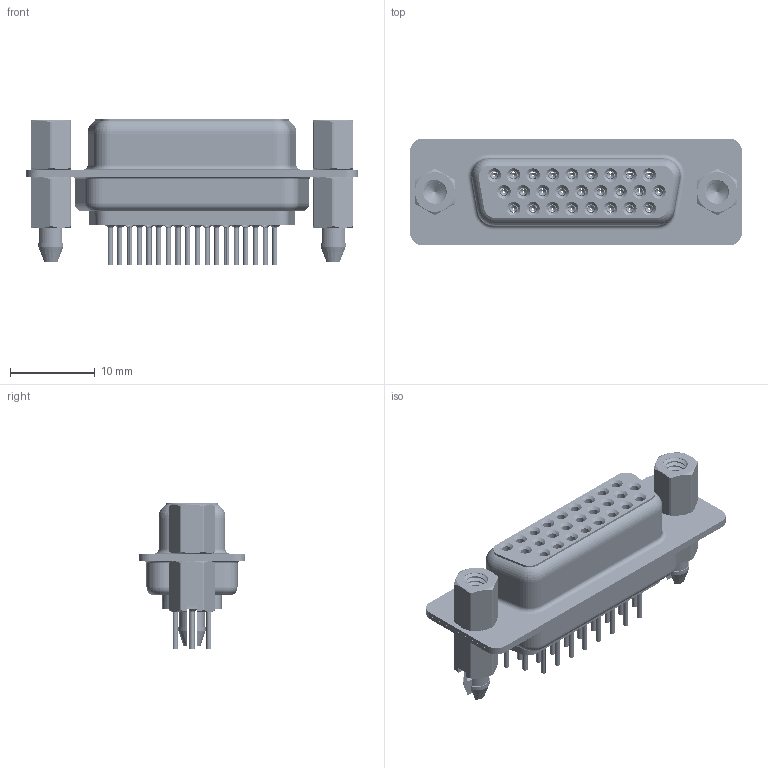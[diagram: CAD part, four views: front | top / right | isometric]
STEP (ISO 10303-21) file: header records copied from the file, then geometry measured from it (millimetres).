
FILE_DESCRIPTION (( 'STEP AP203' ), '1' );
FILE_NAME ('638-026-330-047.STEP', '2020-07-18T20:21:01', ( '' ), ( '' ), 'SwSTEP 2.0', 'SolidWorks 2020', '' );
FILE_SCHEMA (( 'CONFIG_CONTROL_DESIGN' ));
Length unit declared in the file: millimetre
Products named in the file (9): 638 Housing_26 Contacts; 638 Contact Row 3_30; 638 Contact Row 2_30; 638 Contact Row 1_30; 638 Shell Rear_26 Contacts; 638 4-40 Threaded Boardlock_LP; 638-026-330-047; 638 Shell Front_26 Contacts; 638 4-40 Hex Standoff
Assembly tree (33 placements, depth 2):
  638-026-330-047
    638 Housing_26 Contacts
    638 Shell Front_26 Contacts
    638 Shell Rear_26 Contacts
    638 Contact Row 1_30  x9
    638 Contact Row 2_30  x9
    638 Contact Row 3_30  x8
    638 4-40 Hex Standoff  x2
    638 4-40 Threaded Boardlock_LP  x2
Bounding box: 39.19 x 12.6 x 17.3 mm (x, y, z)
Volume: 2538.5 mm3; surface area: 9075.2 mm2
Topology: 33 solids, 33 shells, 3781 faces, 9689 edges, 6035 vertices
Faces by surface type: cylinder 1099, plane 927, torus 733, bspline 538, cone 484
Entity records: 38592 total; most frequent: CARTESIAN_POINT 13129, DIRECTION 5076, ORIENTED_EDGE 4986, EDGE_CURVE 2493, AXIS2_PLACEMENT_3D 2104, VERTEX_POINT 1577, EDGE_LOOP 1174, CIRCLE 1117
